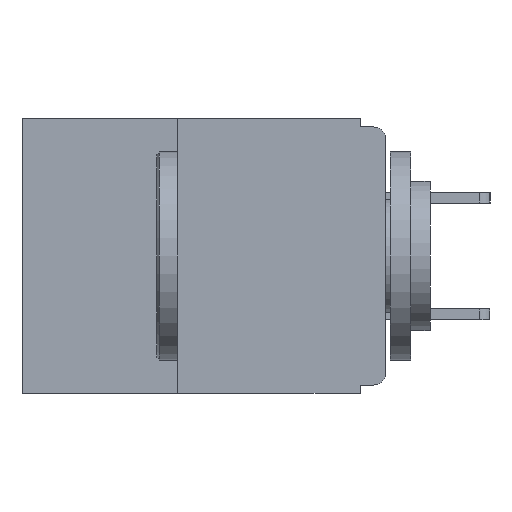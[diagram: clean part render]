
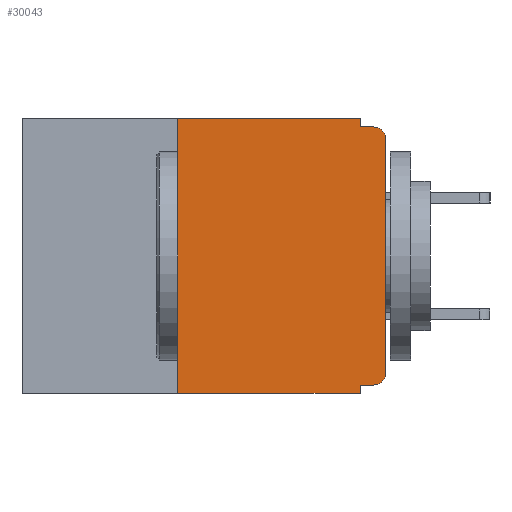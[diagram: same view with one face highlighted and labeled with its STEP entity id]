
A CAD part, left-side view. The second image highlights one B-rep face of the part: STEP entity #30043.
In plain terms, the highlighted planar face has unit normal (-1, 0, 0).
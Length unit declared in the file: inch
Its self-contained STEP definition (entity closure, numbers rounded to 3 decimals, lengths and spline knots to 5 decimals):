
#603 = VERTEX_POINT ( 'NONE', #607 ) ;
#607 = CARTESIAN_POINT ( 'NONE',  ( 0., 0., -0.025 ) ) ;
#830 = VECTOR ( 'NONE', #4927, 39.37008 ) ;
#860 = VECTOR ( 'NONE', #10915, 39.37008 ) ;
#1816 = VERTEX_POINT ( 'NONE', #17304 ) ;
#2175 = DIRECTION ( 'NONE',  ( 0., -1., 0. ) ) ;
#2952 = DIRECTION ( 'NONE',  ( 0., 0., -1. ) ) ;
#3365 = VECTOR ( 'NONE', #4104, 39.37008 ) ;
#3915 = EDGE_CURVE ( 'NONE', #603, #28256, #16452, .T. ) ;
#4104 = DIRECTION ( 'NONE',  ( 0., -1., 0. ) ) ;
#4518 = CARTESIAN_POINT ( 'NONE',  ( 0., 0., -0.01 ) ) ;
#4668 = VERTEX_POINT ( 'NONE', #27094 ) ;
#4927 = DIRECTION ( 'NONE',  ( 0., 1., 0. ) ) ;
#5267 = CARTESIAN_POINT ( 'NONE',  ( 0., 0., -0.32 ) ) ;
#5782 = EDGE_CURVE ( 'NONE', #4668, #26778, #6822, .T. ) ;
#6150 = EDGE_CURVE ( 'NONE', #24567, #10014, #14400, .T. ) ;
#6822 = LINE ( 'NONE', #11362, #860 ) ;
#8477 = EDGE_LOOP ( 'NONE', ( #25455, #26079, #26421, #26483, #26741, #26775, #27294, #27779, #27946, #28471 ) ) ;
#9057 = EDGE_CURVE ( 'NONE', #23149, #28256, #19276, .T. ) ;
#9323 = CARTESIAN_POINT ( 'NONE',  ( 0., 0.015, -0.32 ) ) ;
#10014 = VERTEX_POINT ( 'NONE', #19816 ) ;
#10401 = EDGE_CURVE ( 'NONE', #26778, #15307, #23442, .T. ) ;
#10600 = PLANE ( 'NONE',  #31037 ) ;
#10610 = FACE_OUTER_BOUND ( 'NONE', #8477, .T. ) ;
#10915 = DIRECTION ( 'NONE',  ( 0., 0., 1. ) ) ;
#11270 = DIRECTION ( 'NONE',  ( 0., 0., 1. ) ) ;
#11362 = CARTESIAN_POINT ( 'NONE',  ( 0., 0.25, -0.33 ) ) ;
#12633 = CARTESIAN_POINT ( 'NONE',  ( 0., 0., -0.305 ) ) ;
#13175 = DIRECTION ( 'NONE',  ( 1., 0., 0. ) ) ;
#13205 = LINE ( 'NONE', #15064, #25672 ) ;
#13564 = CARTESIAN_POINT ( 'NONE',  ( 0., 0.015, -0.305 ) ) ;
#14053 = DIRECTION ( 'NONE',  ( 0., -1., 0. ) ) ;
#14163 = CARTESIAN_POINT ( 'NONE',  ( 0., 0.437, 0. ) ) ;
#14400 = LINE ( 'NONE', #5267, #830 ) ;
#14524 = VECTOR ( 'NONE', #11270, 39.37008 ) ;
#15038 = CIRCLE ( 'NONE', #23582, 0.015 ) ;
#15064 = CARTESIAN_POINT ( 'NONE',  ( 0., 0.031, -0.33 ) ) ;
#15307 = VERTEX_POINT ( 'NONE', #30046 ) ;
#16065 = DIRECTION ( 'NONE',  ( 0., 0., -1. ) ) ;
#16452 = CIRCLE ( 'NONE', #23558, 0.015 ) ;
#16814 = VECTOR ( 'NONE', #14053, 39.37008 ) ;
#17304 = CARTESIAN_POINT ( 'NONE',  ( 0., 0.031, -0.33 ) ) ;
#17410 = CARTESIAN_POINT ( 'NONE',  ( 0., 0.437, -0.33 ) ) ;
#17544 = DIRECTION ( 'NONE',  ( 0., 0., -1. ) ) ;
#17581 = DIRECTION ( 'NONE',  ( 0., 0., -1. ) ) ;
#17613 = DIRECTION ( 'NONE',  ( -1., 0., 0. ) ) ;
#17716 = CARTESIAN_POINT ( 'NONE',  ( 0., 0.015, -0.025 ) ) ;
#17784 = CARTESIAN_POINT ( 'NONE',  ( 0., 0.25, 0. ) ) ;
#18441 = EDGE_CURVE ( 'NONE', #4668, #1816, #24875, .T. ) ;
#19276 = LINE ( 'NONE', #4518, #3365 ) ;
#19816 = CARTESIAN_POINT ( 'NONE',  ( 0., 0.031, -0.32 ) ) ;
#20385 = CARTESIAN_POINT ( 'NONE',  ( 0., 0.015, -0.01 ) ) ;
#20605 = EDGE_CURVE ( 'NONE', #24567, #28188, #15038, .T. ) ;
#20705 = CARTESIAN_POINT ( 'NONE',  ( 0., 0.031, 0. ) ) ;
#23149 = VERTEX_POINT ( 'NONE', #27736 ) ;
#23442 = LINE ( 'NONE', #14163, #16814 ) ;
#23558 = AXIS2_PLACEMENT_3D ( 'NONE', #17716, #17613, #17544 ) ;
#23582 = AXIS2_PLACEMENT_3D ( 'NONE', #13564, #30944, #16065 ) ;
#23857 = VECTOR ( 'NONE', #2952, 39.37008 ) ;
#24567 = VERTEX_POINT ( 'NONE', #9323 ) ;
#24875 = LINE ( 'NONE', #17410, #30662 ) ;
#25455 = ORIENTED_EDGE ( 'NONE', *, *, #30746, .T. ) ;
#25584 = EDGE_CURVE ( 'NONE', #15307, #23149, #31192, .T. ) ;
#25672 = VECTOR ( 'NONE', #17581, 39.37008 ) ;
#26079 = ORIENTED_EDGE ( 'NONE', *, *, #3915, .T. ) ;
#26255 = CARTESIAN_POINT ( 'NONE',  ( 0., 0., 0. ) ) ;
#26421 = ORIENTED_EDGE ( 'NONE', *, *, #9057, .F. ) ;
#26483 = ORIENTED_EDGE ( 'NONE', *, *, #25584, .F. ) ;
#26741 = ORIENTED_EDGE ( 'NONE', *, *, #10401, .F. ) ;
#26775 = ORIENTED_EDGE ( 'NONE', *, *, #5782, .F. ) ;
#26778 = VERTEX_POINT ( 'NONE', #17784 ) ;
#27094 = CARTESIAN_POINT ( 'NONE',  ( 0., 0.25, -0.33 ) ) ;
#27294 = ORIENTED_EDGE ( 'NONE', *, *, #18441, .T. ) ;
#27474 = EDGE_CURVE ( 'NONE', #10014, #1816, #13205, .T. ) ;
#27736 = CARTESIAN_POINT ( 'NONE',  ( 0., 0.031, -0.01 ) ) ;
#27779 = ORIENTED_EDGE ( 'NONE', *, *, #27474, .F. ) ;
#27792 = LINE ( 'NONE', #26255, #14524 ) ;
#27946 = ORIENTED_EDGE ( 'NONE', *, *, #6150, .F. ) ;
#28102 = CARTESIAN_POINT ( 'NONE',  ( 0., 0.437, 0. ) ) ;
#28188 = VERTEX_POINT ( 'NONE', #12633 ) ;
#28256 = VERTEX_POINT ( 'NONE', #20385 ) ;
#28471 = ORIENTED_EDGE ( 'NONE', *, *, #20605, .T. ) ;
#30043 = ADVANCED_FACE ( 'NONE', ( #10610 ), #10600, .F. ) ;
#30046 = CARTESIAN_POINT ( 'NONE',  ( 0., 0.031, 0. ) ) ;
#30550 = DIRECTION ( 'NONE',  ( 0., 0., -1. ) ) ;
#30662 = VECTOR ( 'NONE', #2175, 39.37008 ) ;
#30746 = EDGE_CURVE ( 'NONE', #28188, #603, #27792, .T. ) ;
#30944 = DIRECTION ( 'NONE',  ( -1., 0., 0. ) ) ;
#31037 = AXIS2_PLACEMENT_3D ( 'NONE', #28102, #13175, #30550 ) ;
#31192 = LINE ( 'NONE', #20705, #23857 ) ;
